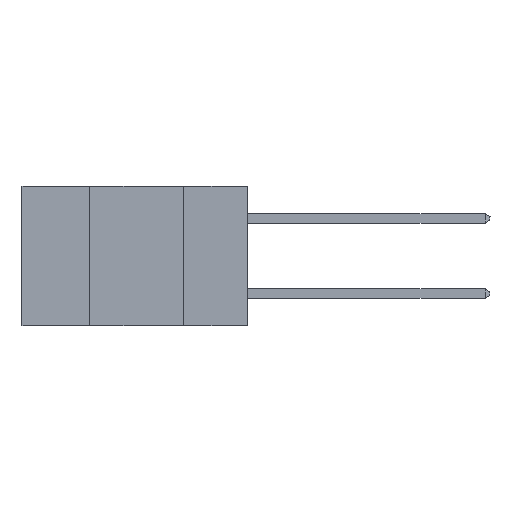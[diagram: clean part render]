
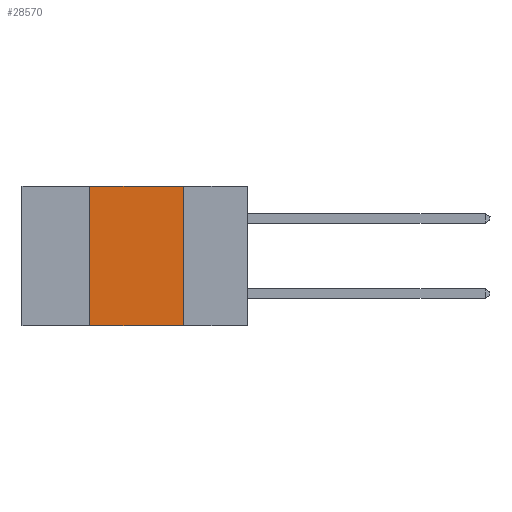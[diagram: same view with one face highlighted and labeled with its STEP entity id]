
A CAD part, left-side view. The second image highlights one B-rep face of the part: STEP entity #28570.
In plain terms, the highlighted planar face has unit normal (-1, 0, 0).
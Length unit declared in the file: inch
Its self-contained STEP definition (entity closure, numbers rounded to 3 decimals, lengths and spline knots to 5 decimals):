
#1533 = VERTEX_POINT ( 'NONE', #8952 ) ;
#1960 = EDGE_LOOP ( 'NONE', ( #21802, #28427, #4663, #3925 ) ) ;
#2073 = EDGE_CURVE ( 'NONE', #18893, #22636, #28846, .T. ) ;
#3052 = DIRECTION ( 'NONE',  ( 1., 0., 0. ) ) ;
#3925 = ORIENTED_EDGE ( 'NONE', *, *, #11191, .T. ) ;
#4558 = FACE_OUTER_BOUND ( 'NONE', #1960, .T. ) ;
#4663 = ORIENTED_EDGE ( 'NONE', *, *, #23731, .F. ) ;
#4925 = DIRECTION ( 'NONE',  ( 0., -1., 0. ) ) ;
#5294 = CARTESIAN_POINT ( 'NONE',  ( 0., 0.17, 0. ) ) ;
#5947 = EDGE_CURVE ( 'NONE', #1533, #18893, #22152, .T. ) ;
#8952 = CARTESIAN_POINT ( 'NONE',  ( 0., 0.42, 0. ) ) ;
#10913 = VECTOR ( 'NONE', #4925, 39.37008 ) ;
#11191 = EDGE_CURVE ( 'NONE', #13937, #22636, #17320, .T. ) ;
#12582 = CARTESIAN_POINT ( 'NONE',  ( 0., 0.17, 0. ) ) ;
#13937 = VERTEX_POINT ( 'NONE', #26447 ) ;
#13968 = LINE ( 'NONE', #25416, #19261 ) ;
#13987 = CARTESIAN_POINT ( 'NONE',  ( 0., 0.6, -0.37 ) ) ;
#14359 = DIRECTION ( 'NONE',  ( 0., 0., 1. ) ) ;
#16258 = DIRECTION ( 'NONE',  ( 0., -1., 0. ) ) ;
#16507 = CARTESIAN_POINT ( 'NONE',  ( 0., 0.6, 0. ) ) ;
#16690 = CARTESIAN_POINT ( 'NONE',  ( 0., 0.6, 0. ) ) ;
#17320 = LINE ( 'NONE', #13987, #28311 ) ;
#18056 = AXIS2_PLACEMENT_3D ( 'NONE', #16507, #3052, #18794 ) ;
#18794 = DIRECTION ( 'NONE',  ( 0., 0., -1. ) ) ;
#18893 = VERTEX_POINT ( 'NONE', #5294 ) ;
#19261 = VECTOR ( 'NONE', #14359, 39.37008 ) ;
#21802 = ORIENTED_EDGE ( 'NONE', *, *, #2073, .F. ) ;
#22152 = LINE ( 'NONE', #16690, #10913 ) ;
#22636 = VERTEX_POINT ( 'NONE', #26754 ) ;
#23085 = VECTOR ( 'NONE', #28123, 39.37008 ) ;
#23731 = EDGE_CURVE ( 'NONE', #13937, #1533, #13968, .T. ) ;
#25203 = PLANE ( 'NONE',  #18056 ) ;
#25416 = CARTESIAN_POINT ( 'NONE',  ( 0., 0.42, 0. ) ) ;
#26447 = CARTESIAN_POINT ( 'NONE',  ( 0., 0.42, -0.37 ) ) ;
#26754 = CARTESIAN_POINT ( 'NONE',  ( 0., 0.17, -0.37 ) ) ;
#28123 = DIRECTION ( 'NONE',  ( 0., 0., -1. ) ) ;
#28311 = VECTOR ( 'NONE', #16258, 39.37008 ) ;
#28427 = ORIENTED_EDGE ( 'NONE', *, *, #5947, .F. ) ;
#28570 = ADVANCED_FACE ( 'NONE', ( #4558 ), #25203, .F. ) ;
#28846 = LINE ( 'NONE', #12582, #23085 ) ;
